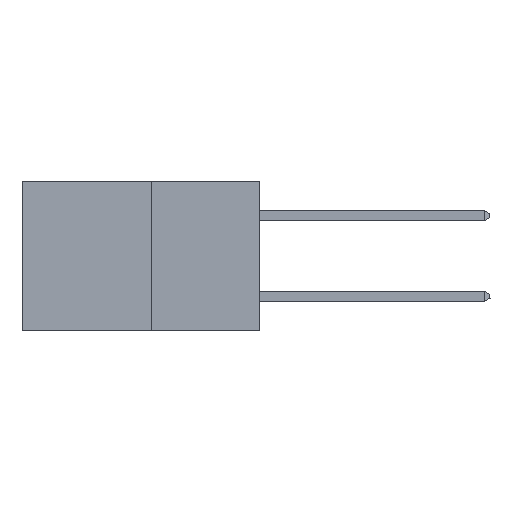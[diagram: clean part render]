
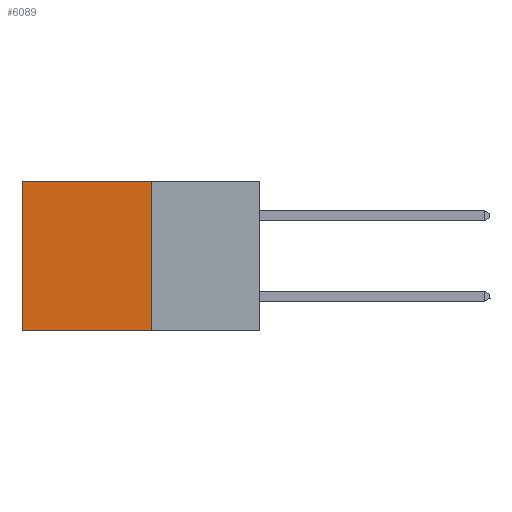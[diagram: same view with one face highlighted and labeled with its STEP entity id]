
A CAD part, left-side view. The second image highlights one B-rep face of the part: STEP entity #6089.
In plain terms, the highlighted planar face has unit normal (-1, 0, 0).
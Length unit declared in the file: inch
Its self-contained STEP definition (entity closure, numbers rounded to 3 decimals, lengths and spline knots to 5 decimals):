
#111 = CARTESIAN_POINT ( 'NONE',  ( 0.277, 0.59, -0.37 ) ) ;
#312 = ORIENTED_EDGE ( 'NONE', *, *, #15094, .F. ) ;
#1037 = VECTOR ( 'NONE', #1153, 39.37008 ) ;
#1153 = DIRECTION ( 'NONE',  ( 0., 1., 0. ) ) ;
#1865 = DIRECTION ( 'NONE',  ( 0., 0., -1. ) ) ;
#4300 = DIRECTION ( 'NONE',  ( 0., 0., -1. ) ) ;
#4308 = CARTESIAN_POINT ( 'NONE',  ( 0.277, 0.27, -0.37 ) ) ;
#4376 = DIRECTION ( 'NONE',  ( 1., 0., 0. ) ) ;
#4403 = LINE ( 'NONE', #111, #18015 ) ;
#4532 = PLANE ( 'NONE',  #16828 ) ;
#4860 = CARTESIAN_POINT ( 'NONE',  ( 0.277, 0.27, -0.37 ) ) ;
#5137 = ORIENTED_EDGE ( 'NONE', *, *, #9383, .T. ) ;
#5754 = LINE ( 'NONE', #8225, #1037 ) ;
#6089 = ADVANCED_FACE ( 'NONE', ( #14661 ), #4532, .F. ) ;
#8225 = CARTESIAN_POINT ( 'NONE',  ( 0.277, 0.27, 0. ) ) ;
#9383 = EDGE_CURVE ( 'NONE', #17565, #17907, #5754, .T. ) ;
#9427 = EDGE_CURVE ( 'NONE', #19091, #21715, #19310, .T. ) ;
#9677 = VECTOR ( 'NONE', #17369, 39.37008 ) ;
#10202 = CARTESIAN_POINT ( 'NONE',  ( 0.277, 0.27, -0.37 ) ) ;
#11871 = DIRECTION ( 'NONE',  ( 0., 1., 0. ) ) ;
#12152 = ORIENTED_EDGE ( 'NONE', *, *, #9427, .F. ) ;
#13113 = CARTESIAN_POINT ( 'NONE',  ( 0.277, 0.59, -0.37 ) ) ;
#14420 = LINE ( 'NONE', #10202, #9677 ) ;
#14661 = FACE_OUTER_BOUND ( 'NONE', #18263, .T. ) ;
#15094 = EDGE_CURVE ( 'NONE', #17565, #19091, #14420, .T. ) ;
#15577 = VECTOR ( 'NONE', #11871, 39.37008 ) ;
#16828 = AXIS2_PLACEMENT_3D ( 'NONE', #4860, #4376, #4300 ) ;
#17369 = DIRECTION ( 'NONE',  ( 0., 0., -1. ) ) ;
#17565 = VERTEX_POINT ( 'NONE', #18410 ) ;
#17907 = VERTEX_POINT ( 'NONE', #22088 ) ;
#18015 = VECTOR ( 'NONE', #1865, 39.37008 ) ;
#18075 = ORIENTED_EDGE ( 'NONE', *, *, #18252, .T. ) ;
#18252 = EDGE_CURVE ( 'NONE', #17907, #21715, #4403, .T. ) ;
#18263 = EDGE_LOOP ( 'NONE', ( #18075, #12152, #312, #5137 ) ) ;
#18410 = CARTESIAN_POINT ( 'NONE',  ( 0.277, 0.27, 0. ) ) ;
#19091 = VERTEX_POINT ( 'NONE', #4308 ) ;
#19310 = LINE ( 'NONE', #22299, #15577 ) ;
#21715 = VERTEX_POINT ( 'NONE', #13113 ) ;
#22088 = CARTESIAN_POINT ( 'NONE',  ( 0.277, 0.59, 0. ) ) ;
#22299 = CARTESIAN_POINT ( 'NONE',  ( 0.277, 0.27, -0.37 ) ) ;
